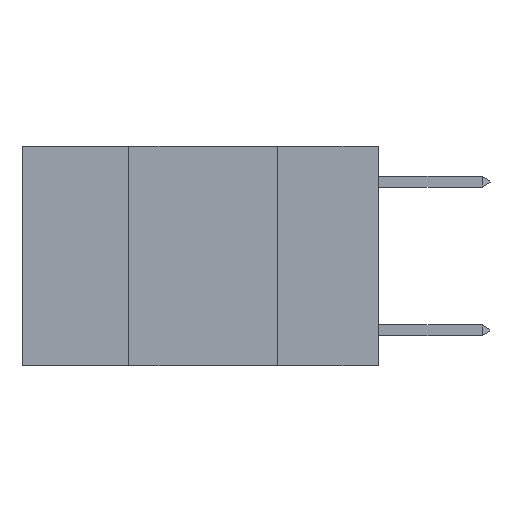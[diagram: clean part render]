
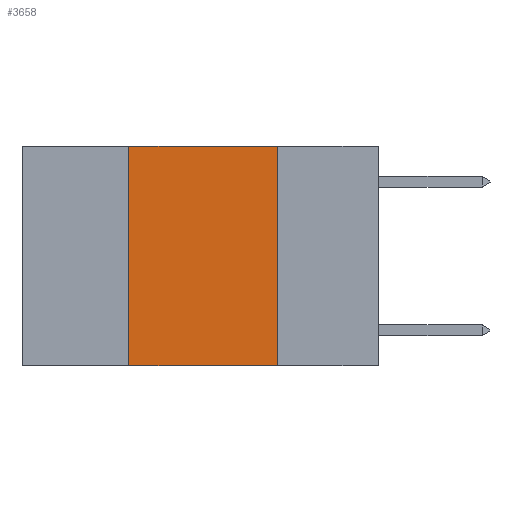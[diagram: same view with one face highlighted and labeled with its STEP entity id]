
A CAD part, left-side view. The second image highlights one B-rep face of the part: STEP entity #3658.
In plain terms, the highlighted planar face has unit normal (-1, 0, 0).
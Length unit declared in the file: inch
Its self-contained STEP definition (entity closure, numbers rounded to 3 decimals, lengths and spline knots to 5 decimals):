
#17 = DIRECTION ( 'NONE',  ( 0., 0., 1. ) ) ;
#88 = CARTESIAN_POINT ( 'NONE',  ( 0., 0.42, 0. ) ) ;
#337 = CARTESIAN_POINT ( 'NONE',  ( 0., 0.6, 0. ) ) ;
#460 = LINE ( 'NONE', #8734, #8407 ) ;
#648 = DIRECTION ( 'NONE',  ( 0., 0., -1. ) ) ;
#892 = CARTESIAN_POINT ( 'NONE',  ( 0., 0.17, -0.37 ) ) ;
#955 = ORIENTED_EDGE ( 'NONE', *, *, #9767, .F. ) ;
#1143 = DIRECTION ( 'NONE',  ( 1., 0., 0. ) ) ;
#1451 = EDGE_CURVE ( 'NONE', #6111, #8205, #5715, .T. ) ;
#2673 = VECTOR ( 'NONE', #3505, 39.37008 ) ;
#2847 = AXIS2_PLACEMENT_3D ( 'NONE', #337, #1143, #6724 ) ;
#3126 = EDGE_CURVE ( 'NONE', #6111, #4749, #4789, .T. ) ;
#3166 = DIRECTION ( 'NONE',  ( 0., -1., 0. ) ) ;
#3404 = ORIENTED_EDGE ( 'NONE', *, *, #3126, .T. ) ;
#3505 = DIRECTION ( 'NONE',  ( 0., -1., 0. ) ) ;
#3658 = ADVANCED_FACE ( 'NONE', ( #4143 ), #9031, .F. ) ;
#4114 = EDGE_CURVE ( 'NONE', #8205, #9692, #460, .T. ) ;
#4143 = FACE_OUTER_BOUND ( 'NONE', #4689, .T. ) ;
#4212 = VECTOR ( 'NONE', #648, 39.37008 ) ;
#4689 = EDGE_LOOP ( 'NONE', ( #955, #8038, #7428, #3404 ) ) ;
#4749 = VERTEX_POINT ( 'NONE', #892 ) ;
#4777 = CARTESIAN_POINT ( 'NONE',  ( 0., 0.42, 0. ) ) ;
#4789 = LINE ( 'NONE', #5097, #2673 ) ;
#5097 = CARTESIAN_POINT ( 'NONE',  ( 0., 0.6, -0.37 ) ) ;
#5276 = CARTESIAN_POINT ( 'NONE',  ( 0., 0.17, 0. ) ) ;
#5416 = CARTESIAN_POINT ( 'NONE',  ( 0., 0.17, 0. ) ) ;
#5466 = VECTOR ( 'NONE', #17, 39.37008 ) ;
#5715 = LINE ( 'NONE', #4777, #5466 ) ;
#6111 = VERTEX_POINT ( 'NONE', #9065 ) ;
#6133 = LINE ( 'NONE', #5416, #4212 ) ;
#6724 = DIRECTION ( 'NONE',  ( 0., 0., -1. ) ) ;
#7428 = ORIENTED_EDGE ( 'NONE', *, *, #1451, .F. ) ;
#8038 = ORIENTED_EDGE ( 'NONE', *, *, #4114, .F. ) ;
#8205 = VERTEX_POINT ( 'NONE', #88 ) ;
#8407 = VECTOR ( 'NONE', #3166, 39.37008 ) ;
#8734 = CARTESIAN_POINT ( 'NONE',  ( 0., 0.6, 0. ) ) ;
#9031 = PLANE ( 'NONE',  #2847 ) ;
#9065 = CARTESIAN_POINT ( 'NONE',  ( 0., 0.42, -0.37 ) ) ;
#9692 = VERTEX_POINT ( 'NONE', #5276 ) ;
#9767 = EDGE_CURVE ( 'NONE', #9692, #4749, #6133, .T. ) ;
